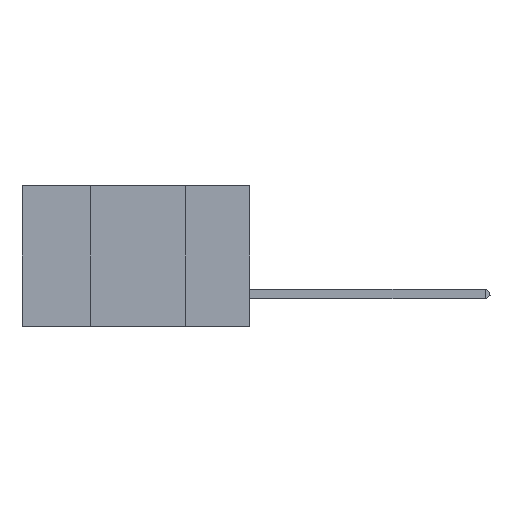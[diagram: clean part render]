
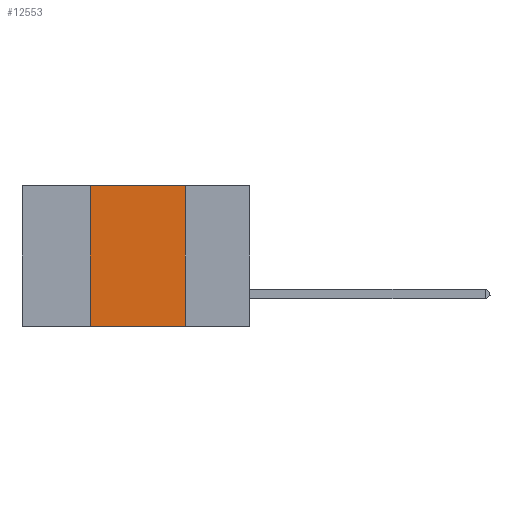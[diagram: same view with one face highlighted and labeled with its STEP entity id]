
A CAD part, left-side view. The second image highlights one B-rep face of the part: STEP entity #12553.
In plain terms, the highlighted planar face has unit normal (-1, 0, 0).
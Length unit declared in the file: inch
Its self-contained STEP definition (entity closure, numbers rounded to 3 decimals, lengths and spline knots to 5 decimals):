
#1318 = EDGE_CURVE ( 'NONE', #19913, #8359, #3724, .T. ) ;
#2391 = VECTOR ( 'NONE', #24018, 39.37008 ) ;
#2948 = ORIENTED_EDGE ( 'NONE', *, *, #31664, .F. ) ;
#3618 = EDGE_LOOP ( 'NONE', ( #2948, #26934, #50069, #37573 ) ) ;
#3724 = LINE ( 'NONE', #50207, #19934 ) ;
#4848 = VECTOR ( 'NONE', #43647, 39.37008 ) ;
#5881 = AXIS2_PLACEMENT_3D ( 'NONE', #46059, #10396, #15282 ) ;
#7812 = CARTESIAN_POINT ( 'NONE',  ( 0., 0.6, -0.37 ) ) ;
#8359 = VERTEX_POINT ( 'NONE', #20668 ) ;
#8462 = CARTESIAN_POINT ( 'NONE',  ( 0., 0.42, -0.37 ) ) ;
#10396 = DIRECTION ( 'NONE',  ( 1., 0., 0. ) ) ;
#12553 = ADVANCED_FACE ( 'NONE', ( #27319 ), #49842, .F. ) ;
#13025 = CARTESIAN_POINT ( 'NONE',  ( 0., 0.17, 0. ) ) ;
#14623 = DIRECTION ( 'NONE',  ( 0., 0., 1. ) ) ;
#15282 = DIRECTION ( 'NONE',  ( 0., 0., -1. ) ) ;
#16071 = LINE ( 'NONE', #32499, #2391 ) ;
#17455 = EDGE_CURVE ( 'NONE', #19913, #17688, #36625, .T. ) ;
#17505 = VERTEX_POINT ( 'NONE', #13025 ) ;
#17688 = VERTEX_POINT ( 'NONE', #49648 ) ;
#19913 = VERTEX_POINT ( 'NONE', #8462 ) ;
#19934 = VECTOR ( 'NONE', #14623, 39.37008 ) ;
#20668 = CARTESIAN_POINT ( 'NONE',  ( 0., 0.42, 0. ) ) ;
#24018 = DIRECTION ( 'NONE',  ( 0., -1., 0. ) ) ;
#26934 = ORIENTED_EDGE ( 'NONE', *, *, #48804, .F. ) ;
#27319 = FACE_OUTER_BOUND ( 'NONE', #3618, .T. ) ;
#31664 = EDGE_CURVE ( 'NONE', #17505, #17688, #32578, .T. ) ;
#32499 = CARTESIAN_POINT ( 'NONE',  ( 0., 0.6, 0. ) ) ;
#32578 = LINE ( 'NONE', #45019, #45626 ) ;
#36625 = LINE ( 'NONE', #7812, #4848 ) ;
#37573 = ORIENTED_EDGE ( 'NONE', *, *, #17455, .T. ) ;
#43647 = DIRECTION ( 'NONE',  ( 0., -1., 0. ) ) ;
#45019 = CARTESIAN_POINT ( 'NONE',  ( 0., 0.17, 0. ) ) ;
#45626 = VECTOR ( 'NONE', #49151, 39.37008 ) ;
#46059 = CARTESIAN_POINT ( 'NONE',  ( 0., 0.6, 0. ) ) ;
#48804 = EDGE_CURVE ( 'NONE', #8359, #17505, #16071, .T. ) ;
#49151 = DIRECTION ( 'NONE',  ( 0., 0., -1. ) ) ;
#49648 = CARTESIAN_POINT ( 'NONE',  ( 0., 0.17, -0.37 ) ) ;
#49842 = PLANE ( 'NONE',  #5881 ) ;
#50069 = ORIENTED_EDGE ( 'NONE', *, *, #1318, .F. ) ;
#50207 = CARTESIAN_POINT ( 'NONE',  ( 0., 0.42, 0. ) ) ;
